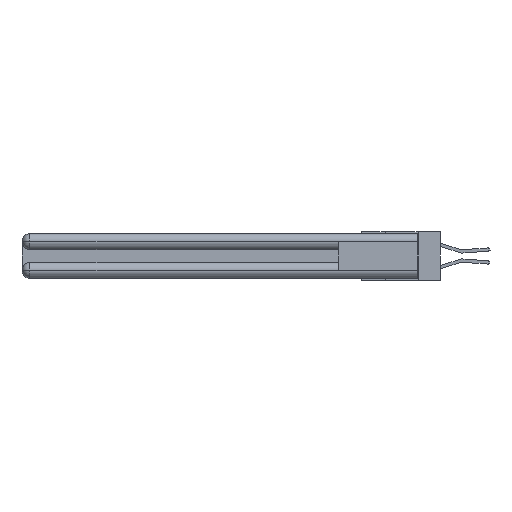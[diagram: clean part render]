
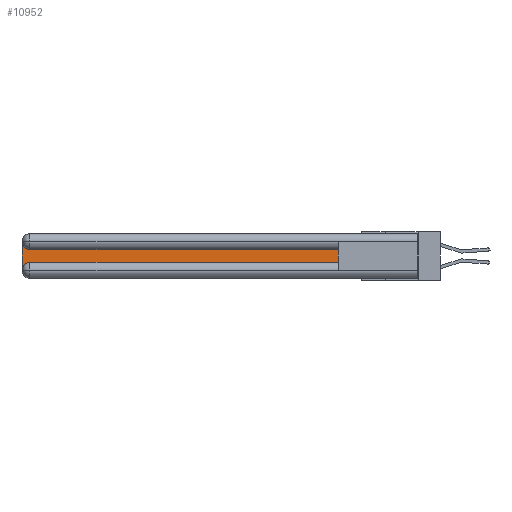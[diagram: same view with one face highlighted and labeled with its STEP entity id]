
A CAD part, left-side view. The second image highlights one B-rep face of the part: STEP entity #10952.
In plain terms, the highlighted planar face has unit normal (-1, 0, 0).
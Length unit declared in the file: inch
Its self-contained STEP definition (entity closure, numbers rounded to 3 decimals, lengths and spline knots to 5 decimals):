
#1505 = LINE ( 'NONE', #32931, #31069 ) ;
#1602 = EDGE_CURVE ( 'NONE', #25591, #20670, #21651, .T. ) ;
#2414 = AXIS2_PLACEMENT_3D ( 'NONE', #11983, #25993, #25635 ) ;
#2835 = VERTEX_POINT ( 'NONE', #14109 ) ;
#3767 = CARTESIAN_POINT ( 'NONE',  ( 0.075, 3., -0.0625 ) ) ;
#4281 = DIRECTION ( 'NONE',  ( 1., 0., 0. ) ) ;
#4860 = ORIENTED_EDGE ( 'NONE', *, *, #15105, .T. ) ;
#4885 = FACE_OUTER_BOUND ( 'NONE', #14295, .T. ) ;
#5026 = AXIS2_PLACEMENT_3D ( 'NONE', #26501, #4281, #7105 ) ;
#5171 = EDGE_CURVE ( 'NONE', #6223, #25591, #19981, .T. ) ;
#5885 = ORIENTED_EDGE ( 'NONE', *, *, #1602, .T. ) ;
#6223 = VERTEX_POINT ( 'NONE', #3767 ) ;
#6925 = CARTESIAN_POINT ( 'NONE',  ( 0.075, 3., -0.2175 ) ) ;
#7105 = DIRECTION ( 'NONE',  ( 0., 0., -1. ) ) ;
#10143 = EDGE_CURVE ( 'NONE', #2835, #6223, #12266, .T. ) ;
#10364 = ORIENTED_EDGE ( 'NONE', *, *, #5171, .T. ) ;
#10952 = ADVANCED_FACE ( 'NONE', ( #4885 ), #25880, .F. ) ;
#11983 = CARTESIAN_POINT ( 'NONE',  ( 0.075, 3., -0.1225 ) ) ;
#12266 = CIRCLE ( 'NONE', #27513, 0.06 ) ;
#12616 = VECTOR ( 'NONE', #29340, 39.37008 ) ;
#13243 = CARTESIAN_POINT ( 'NONE',  ( 0.075, 2.94, -0.0625 ) ) ;
#13609 = CARTESIAN_POINT ( 'NONE',  ( 0.075, 0.6, -0.1225 ) ) ;
#13781 = ORIENTED_EDGE ( 'NONE', *, *, #25534, .T. ) ;
#13946 = DIRECTION ( 'NONE',  ( 0., 0., 1. ) ) ;
#14109 = CARTESIAN_POINT ( 'NONE',  ( 0.075, 2.94, -0.1225 ) ) ;
#14295 = EDGE_LOOP ( 'NONE', ( #25622, #28311, #10364, #5885, #4860, #13781 ) ) ;
#14361 = VECTOR ( 'NONE', #33075, 39.37008 ) ;
#14596 = CARTESIAN_POINT ( 'NONE',  ( 0.075, 2.94, -0.2175 ) ) ;
#15105 = EDGE_CURVE ( 'NONE', #20670, #19985, #18146, .T. ) ;
#18146 = LINE ( 'NONE', #24439, #23778 ) ;
#18752 = CARTESIAN_POINT ( 'NONE',  ( 0.075, 0.6, -0.1225 ) ) ;
#19080 = CARTESIAN_POINT ( 'NONE',  ( 0.075, 3., -0.2775 ) ) ;
#19550 = LINE ( 'NONE', #13609, #14361 ) ;
#19981 = LINE ( 'NONE', #6925, #12616 ) ;
#19985 = VERTEX_POINT ( 'NONE', #22898 ) ;
#20670 = VERTEX_POINT ( 'NONE', #14596 ) ;
#21651 = CIRCLE ( 'NONE', #5026, 0.06 ) ;
#21719 = DIRECTION ( 'NONE',  ( 1., 0., 0. ) ) ;
#22145 = DIRECTION ( 'NONE',  ( 0., -1., 0. ) ) ;
#22898 = CARTESIAN_POINT ( 'NONE',  ( 0.075, 0.6, -0.2175 ) ) ;
#23778 = VECTOR ( 'NONE', #22145, 39.37008 ) ;
#24439 = CARTESIAN_POINT ( 'NONE',  ( 0.075, 0.6, -0.2175 ) ) ;
#25534 = EDGE_CURVE ( 'NONE', #19985, #29014, #1505, .T. ) ;
#25591 = VERTEX_POINT ( 'NONE', #19080 ) ;
#25622 = ORIENTED_EDGE ( 'NONE', *, *, #32198, .T. ) ;
#25635 = DIRECTION ( 'NONE',  ( 0., 0., -1. ) ) ;
#25880 = PLANE ( 'NONE',  #2414 ) ;
#25993 = DIRECTION ( 'NONE',  ( 1., 0., 0. ) ) ;
#26501 = CARTESIAN_POINT ( 'NONE',  ( 0.075, 2.94, -0.2775 ) ) ;
#27513 = AXIS2_PLACEMENT_3D ( 'NONE', #13243, #21719, #29948 ) ;
#28311 = ORIENTED_EDGE ( 'NONE', *, *, #10143, .T. ) ;
#29014 = VERTEX_POINT ( 'NONE', #18752 ) ;
#29340 = DIRECTION ( 'NONE',  ( 0., 0., -1. ) ) ;
#29948 = DIRECTION ( 'NONE',  ( 0., 0., -1. ) ) ;
#31069 = VECTOR ( 'NONE', #13946, 39.37008 ) ;
#32198 = EDGE_CURVE ( 'NONE', #29014, #2835, #19550, .T. ) ;
#32931 = CARTESIAN_POINT ( 'NONE',  ( 0.075, 0.6, -0.2175 ) ) ;
#33075 = DIRECTION ( 'NONE',  ( 0., 1., 0. ) ) ;
